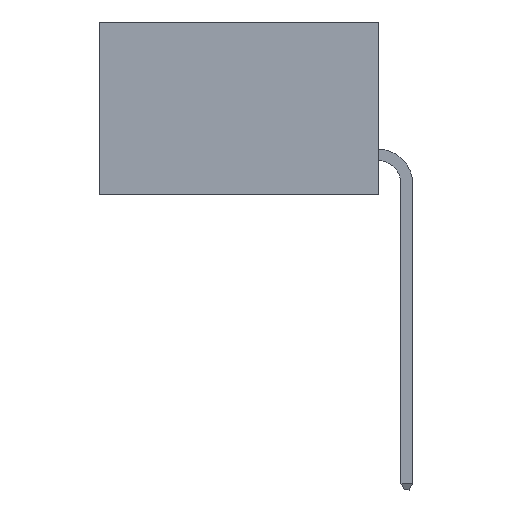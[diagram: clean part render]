
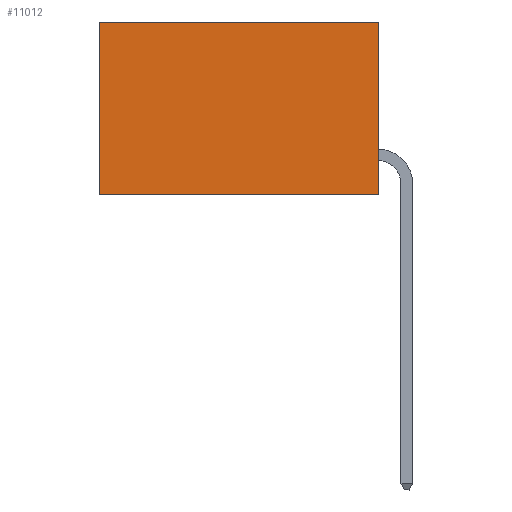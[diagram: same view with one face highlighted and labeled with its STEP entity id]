
A CAD part, left-side view. The second image highlights one B-rep face of the part: STEP entity #11012.
In plain terms, the highlighted planar face has unit normal (-1, 0, 0).
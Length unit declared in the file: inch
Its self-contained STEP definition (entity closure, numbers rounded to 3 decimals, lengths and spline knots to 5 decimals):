
#83 = AXIS2_PLACEMENT_3D ( 'NONE', #5470, #13552, #5167 ) ;
#495 = LINE ( 'NONE', #13566, #2851 ) ;
#1297 = CARTESIAN_POINT ( 'NONE',  ( 0.2615, 0., 0. ) ) ;
#1460 = CARTESIAN_POINT ( 'NONE',  ( 0.2615, 0.6, -0.37 ) ) ;
#1482 = ORIENTED_EDGE ( 'NONE', *, *, #14125, .T. ) ;
#1877 = FACE_OUTER_BOUND ( 'NONE', #9010, .T. ) ;
#2176 = VERTEX_POINT ( 'NONE', #1297 ) ;
#2645 = DIRECTION ( 'NONE',  ( 0., 0., -1. ) ) ;
#2851 = VECTOR ( 'NONE', #13409, 39.37008 ) ;
#3911 = VERTEX_POINT ( 'NONE', #12312 ) ;
#4669 = ORIENTED_EDGE ( 'NONE', *, *, #11230, .F. ) ;
#4686 = VERTEX_POINT ( 'NONE', #9721 ) ;
#4690 = DIRECTION ( 'NONE',  ( 0., 1., 0. ) ) ;
#4744 = EDGE_CURVE ( 'NONE', #2176, #3911, #7403, .T. ) ;
#5167 = DIRECTION ( 'NONE',  ( 0., 0., -1. ) ) ;
#5470 = CARTESIAN_POINT ( 'NONE',  ( 0.2615, 0., -0.37 ) ) ;
#6175 = LINE ( 'NONE', #1460, #7365 ) ;
#7083 = VECTOR ( 'NONE', #2645, 39.37008 ) ;
#7256 = LINE ( 'NONE', #14157, #13481 ) ;
#7365 = VECTOR ( 'NONE', #11035, 39.37008 ) ;
#7403 = LINE ( 'NONE', #14319, #7083 ) ;
#7586 = CARTESIAN_POINT ( 'NONE',  ( 0.2615, 0.6, -0.37 ) ) ;
#8724 = PLANE ( 'NONE',  #83 ) ;
#9010 = EDGE_LOOP ( 'NONE', ( #1482, #4669, #11359, #13813 ) ) ;
#9721 = CARTESIAN_POINT ( 'NONE',  ( 0.2615, 0.6, 0. ) ) ;
#10381 = VERTEX_POINT ( 'NONE', #7586 ) ;
#11012 = ADVANCED_FACE ( 'NONE', ( #1877 ), #8724, .F. ) ;
#11035 = DIRECTION ( 'NONE',  ( 0., 0., -1. ) ) ;
#11230 = EDGE_CURVE ( 'NONE', #3911, #10381, #7256, .T. ) ;
#11359 = ORIENTED_EDGE ( 'NONE', *, *, #4744, .F. ) ;
#12312 = CARTESIAN_POINT ( 'NONE',  ( 0.2615, 0., -0.37 ) ) ;
#13409 = DIRECTION ( 'NONE',  ( 0., 1., 0. ) ) ;
#13481 = VECTOR ( 'NONE', #4690, 39.37008 ) ;
#13552 = DIRECTION ( 'NONE',  ( 1., 0., 0. ) ) ;
#13566 = CARTESIAN_POINT ( 'NONE',  ( 0.2615, 0., 0. ) ) ;
#13687 = EDGE_CURVE ( 'NONE', #2176, #4686, #495, .T. ) ;
#13813 = ORIENTED_EDGE ( 'NONE', *, *, #13687, .T. ) ;
#14125 = EDGE_CURVE ( 'NONE', #4686, #10381, #6175, .T. ) ;
#14157 = CARTESIAN_POINT ( 'NONE',  ( 0.2615, 0., -0.37 ) ) ;
#14319 = CARTESIAN_POINT ( 'NONE',  ( 0.2615, 0., -0.37 ) ) ;
